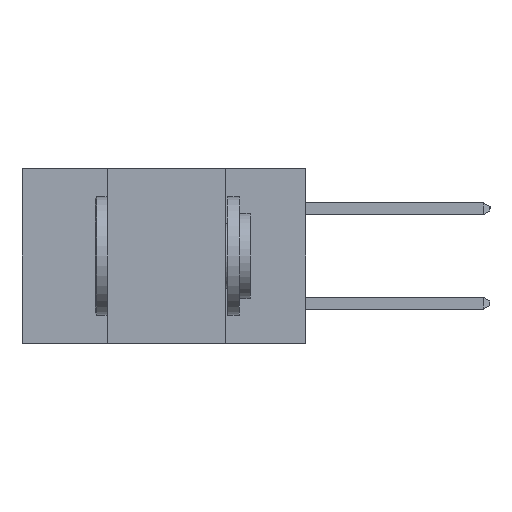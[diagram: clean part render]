
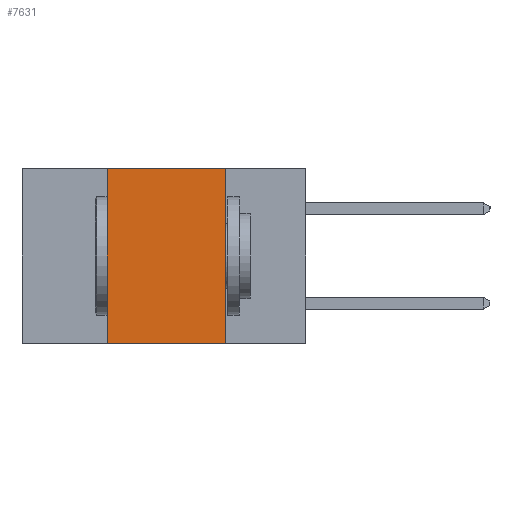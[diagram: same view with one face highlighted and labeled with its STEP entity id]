
A CAD part, left-side view. The second image highlights one B-rep face of the part: STEP entity #7631.
In plain terms, the highlighted planar face has unit normal (-1, 0, 0).
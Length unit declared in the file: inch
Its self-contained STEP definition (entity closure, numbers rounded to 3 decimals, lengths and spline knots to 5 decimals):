
#24 = VERTEX_POINT ( 'NONE', #8459 ) ;
#90 = VECTOR ( 'NONE', #1607, 39.37008 ) ;
#95 = DIRECTION ( 'NONE',  ( 1., 0., 0. ) ) ;
#666 = LINE ( 'NONE', #1351, #4943 ) ;
#735 = DIRECTION ( 'NONE',  ( 0., -1., 0. ) ) ;
#750 = VERTEX_POINT ( 'NONE', #1130 ) ;
#1089 = DIRECTION ( 'NONE',  ( 0., 0., -1. ) ) ;
#1130 = CARTESIAN_POINT ( 'NONE',  ( 0., 0.42, 0. ) ) ;
#1351 = CARTESIAN_POINT ( 'NONE',  ( 0., 0.17, -0.37 ) ) ;
#1607 = DIRECTION ( 'NONE',  ( 0., 0., 1. ) ) ;
#2470 = ORIENTED_EDGE ( 'NONE', *, *, #6497, .F. ) ;
#2624 = VERTEX_POINT ( 'NONE', #5915 ) ;
#2756 = EDGE_CURVE ( 'NONE', #750, #24, #4571, .T. ) ;
#3149 = VECTOR ( 'NONE', #9214, 39.37008 ) ;
#4088 = CARTESIAN_POINT ( 'NONE',  ( 0., 0.42, -0.37 ) ) ;
#4193 = FACE_OUTER_BOUND ( 'NONE', #9386, .T. ) ;
#4571 = LINE ( 'NONE', #7759, #3149 ) ;
#4751 = CARTESIAN_POINT ( 'NONE',  ( 0., 0.6, -0.37 ) ) ;
#4943 = VECTOR ( 'NONE', #6995, 39.37008 ) ;
#5284 = ORIENTED_EDGE ( 'NONE', *, *, #2756, .F. ) ;
#5844 = PLANE ( 'NONE',  #8612 ) ;
#5915 = CARTESIAN_POINT ( 'NONE',  ( 0., 0.17, -0.37 ) ) ;
#6006 = EDGE_CURVE ( 'NONE', #24, #2624, #666, .T. ) ;
#6497 = EDGE_CURVE ( 'NONE', #8988, #750, #6516, .T. ) ;
#6516 = LINE ( 'NONE', #7356, #90 ) ;
#6675 = ORIENTED_EDGE ( 'NONE', *, *, #7402, .T. ) ;
#6995 = DIRECTION ( 'NONE',  ( 0., 0., -1. ) ) ;
#7356 = CARTESIAN_POINT ( 'NONE',  ( 0., 0.42, -0.37 ) ) ;
#7402 = EDGE_CURVE ( 'NONE', #8988, #2624, #7889, .T. ) ;
#7478 = CARTESIAN_POINT ( 'NONE',  ( 0., 0.6, 0. ) ) ;
#7592 = VECTOR ( 'NONE', #735, 39.37008 ) ;
#7631 = ADVANCED_FACE ( 'NONE', ( #4193 ), #5844, .F. ) ;
#7759 = CARTESIAN_POINT ( 'NONE',  ( 0., 0.6, 0. ) ) ;
#7889 = LINE ( 'NONE', #4751, #7592 ) ;
#8459 = CARTESIAN_POINT ( 'NONE',  ( 0., 0.17, 0. ) ) ;
#8612 = AXIS2_PLACEMENT_3D ( 'NONE', #7478, #95, #1089 ) ;
#8988 = VERTEX_POINT ( 'NONE', #4088 ) ;
#9214 = DIRECTION ( 'NONE',  ( 0., -1., 0. ) ) ;
#9386 = EDGE_LOOP ( 'NONE', ( #10179, #5284, #2470, #6675 ) ) ;
#10179 = ORIENTED_EDGE ( 'NONE', *, *, #6006, .F. ) ;
